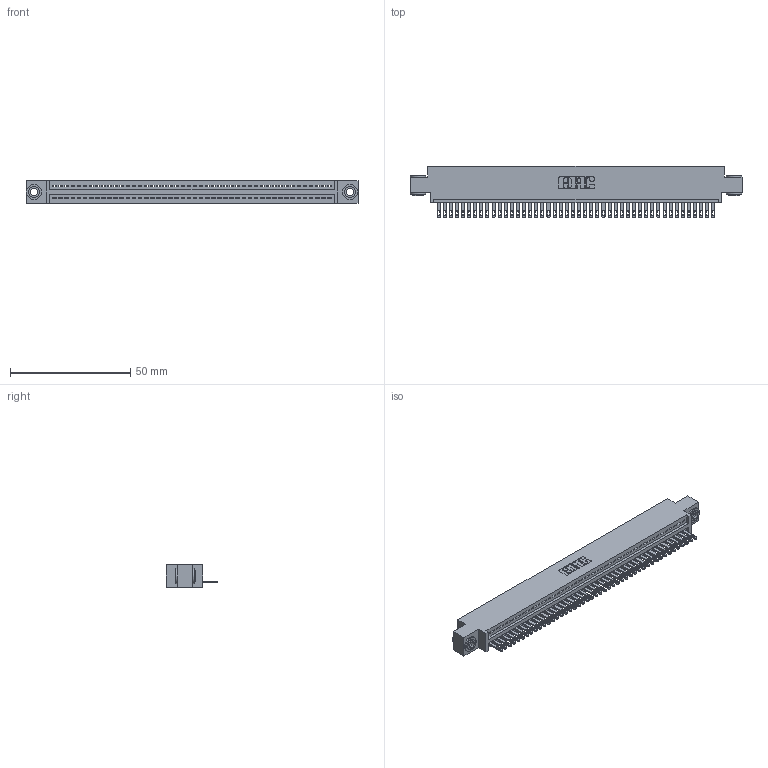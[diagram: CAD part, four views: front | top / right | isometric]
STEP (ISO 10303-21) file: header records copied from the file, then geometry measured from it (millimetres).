
FILE_DESCRIPTION (( 'STEP AP203' ), '1' );
FILE_NAME ('895-046-500-603.STEP', '2020-09-27T04:59:30', ( '' ), ( '' ), 'SwSTEP 2.0', 'SolidWorks 2020', '' );
FILE_SCHEMA (( 'CONFIG_CONTROL_DESIGN' ));
Length unit declared in the file: inch
Products named in the file (4): 895-046-500-603; 845 Part_0.170 Offset - 0.156 Dia-TH; 345-292-001_345-293-100; 345-250-002_345-250-002-102
Assembly tree (49 placements, depth 2):
  895-046-500-603
    845 Part_0.170 Offset - 0.156 Dia-TH
    345-292-001_345-293-100  x46
    345-250-002_345-250-002-102  x2
Bounding box: 138.05 x 21.51 x 9.4 mm (x, y, z)
Volume: 13079.3 mm3; surface area: 17879.9 mm2
Topology: 49 solids, 49 shells, 2652 faces, 8157 edges, 5434 vertices
Faces by surface type: plane 1658, cylinder 986, cone 8
Entity records: 34794 total; most frequent: CARTESIAN_POINT 6005, ORIENTED_EDGE 5978, DIRECTION 5271, EDGE_CURVE 2989, LINE 2645, VECTOR 2645, VERTEX_POINT 1990, AXIS2_PLACEMENT_3D 1313
